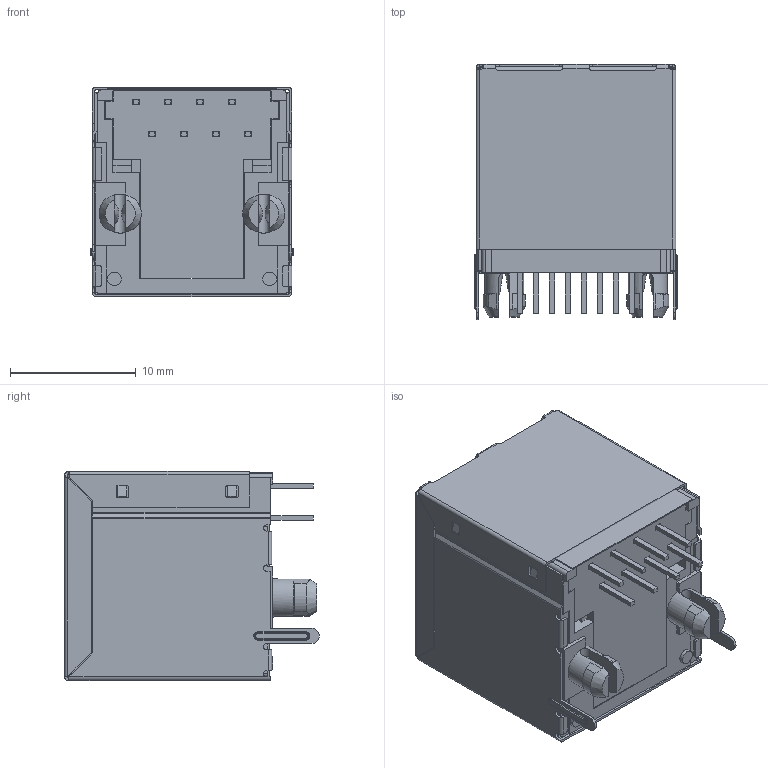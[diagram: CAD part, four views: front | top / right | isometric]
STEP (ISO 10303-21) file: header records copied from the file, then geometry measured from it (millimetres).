
FILE_DESCRIPTION (( 'STEP AP203' ), '1' );
FILE_NAME ('RJ2L018831P00831.STEP', '2019-12-16T14:17:14', ( '' ), ( '' ), 'SwSTEP 2.0', 'SolidWorks 2016', '' );
FILE_SCHEMA (( 'CONFIG_CONTROL_DESIGN' ));
Length unit declared in the file: millimetre
Products named in the file (6): 2L Insulator; 2L Mylar Tape; RJ2L018831P00831; 2L Contacts; 2L Contact Lock; 2L Shield
Assembly tree (5 placements, depth 2):
  RJ2L018831P00831
    2L Insulator
    2L Contacts
    2L Contact Lock
    2L Mylar Tape
    2L Shield
Bounding box: 16.2 x 20.3 x 16.65 mm (x, y, z)
Volume: 2735.3 mm3; surface area: 6842.7 mm2
Topology: 12 solids, 12 shells, 1131 faces, 3180 edges, 2051 vertices
Faces by surface type: plane 784, cylinder 284, bspline 55, cone 8
Entity records: 38238 total; most frequent: CARTESIAN_POINT 9139, ORIENTED_EDGE 6344, DIRECTION 5349, EDGE_CURVE 3172, LINE 2455, VECTOR 2455, VERTEX_POINT 2051, AXIS2_PLACEMENT_3D 1447
